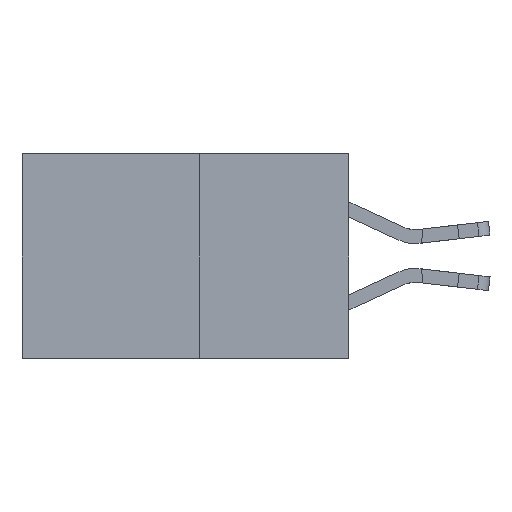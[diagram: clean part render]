
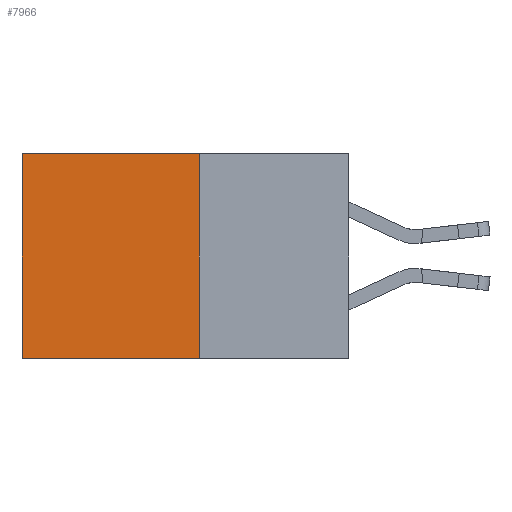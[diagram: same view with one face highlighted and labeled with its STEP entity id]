
A CAD part, left-side view. The second image highlights one B-rep face of the part: STEP entity #7966.
In plain terms, the highlighted planar face has unit normal (-1, 0, 0).
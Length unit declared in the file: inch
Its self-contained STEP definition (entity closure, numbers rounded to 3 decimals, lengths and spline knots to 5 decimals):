
#559 = CARTESIAN_POINT ( 'NONE',  ( 0.277, 0.27, -0.37 ) ) ;
#1659 = ORIENTED_EDGE ( 'NONE', *, *, #14455, .T. ) ;
#1801 = EDGE_LOOP ( 'NONE', ( #1659, #14163, #24694, #23273 ) ) ;
#1871 = FACE_OUTER_BOUND ( 'NONE', #1801, .T. ) ;
#1873 = CARTESIAN_POINT ( 'NONE',  ( 0.277, 0.27, -0.37 ) ) ;
#2361 = AXIS2_PLACEMENT_3D ( 'NONE', #18152, #8397, #22075 ) ;
#3646 = CARTESIAN_POINT ( 'NONE',  ( 0.277, 0.59, -0.37 ) ) ;
#4087 = LINE ( 'NONE', #16967, #8708 ) ;
#4219 = LINE ( 'NONE', #559, #14075 ) ;
#7742 = VECTOR ( 'NONE', #17585, 39.37008 ) ;
#7966 = ADVANCED_FACE ( 'NONE', ( #1871 ), #20139, .F. ) ;
#8397 = DIRECTION ( 'NONE',  ( 1., 0., 0. ) ) ;
#8439 = DIRECTION ( 'NONE',  ( 0., 0., -1. ) ) ;
#8705 = LINE ( 'NONE', #17060, #24870 ) ;
#8708 = VECTOR ( 'NONE', #22837, 39.37008 ) ;
#10011 = VERTEX_POINT ( 'NONE', #10827 ) ;
#10827 = CARTESIAN_POINT ( 'NONE',  ( 0.277, 0.27, 0. ) ) ;
#11336 = CARTESIAN_POINT ( 'NONE',  ( 0.277, 0.27, -0.37 ) ) ;
#14075 = VECTOR ( 'NONE', #8439, 39.37008 ) ;
#14163 = ORIENTED_EDGE ( 'NONE', *, *, #15886, .F. ) ;
#14455 = EDGE_CURVE ( 'NONE', #19064, #17083, #4087, .T. ) ;
#15886 = EDGE_CURVE ( 'NONE', #16263, #17083, #22986, .T. ) ;
#16263 = VERTEX_POINT ( 'NONE', #11336 ) ;
#16775 = CARTESIAN_POINT ( 'NONE',  ( 0.277, 0.59, 0. ) ) ;
#16967 = CARTESIAN_POINT ( 'NONE',  ( 0.277, 0.59, -0.37 ) ) ;
#17060 = CARTESIAN_POINT ( 'NONE',  ( 0.277, 0.27, 0. ) ) ;
#17083 = VERTEX_POINT ( 'NONE', #3646 ) ;
#17585 = DIRECTION ( 'NONE',  ( 0., 1., 0. ) ) ;
#18152 = CARTESIAN_POINT ( 'NONE',  ( 0.277, 0.27, -0.37 ) ) ;
#19031 = DIRECTION ( 'NONE',  ( 0., 1., 0. ) ) ;
#19064 = VERTEX_POINT ( 'NONE', #16775 ) ;
#19656 = EDGE_CURVE ( 'NONE', #10011, #16263, #4219, .T. ) ;
#20139 = PLANE ( 'NONE',  #2361 ) ;
#21959 = EDGE_CURVE ( 'NONE', #10011, #19064, #8705, .T. ) ;
#22075 = DIRECTION ( 'NONE',  ( 0., 0., -1. ) ) ;
#22837 = DIRECTION ( 'NONE',  ( 0., 0., -1. ) ) ;
#22986 = LINE ( 'NONE', #1873, #7742 ) ;
#23273 = ORIENTED_EDGE ( 'NONE', *, *, #21959, .T. ) ;
#24694 = ORIENTED_EDGE ( 'NONE', *, *, #19656, .F. ) ;
#24870 = VECTOR ( 'NONE', #19031, 39.37008 ) ;
